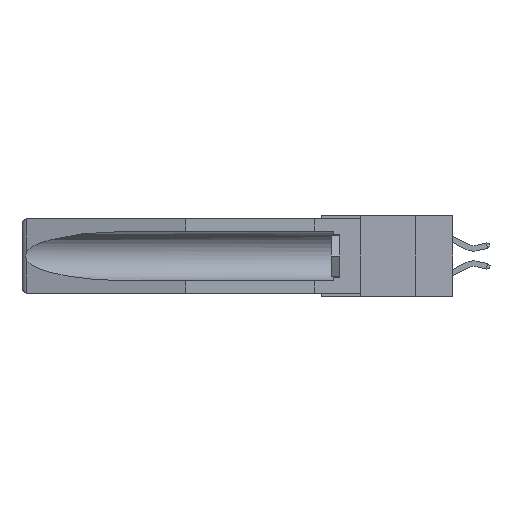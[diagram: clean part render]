
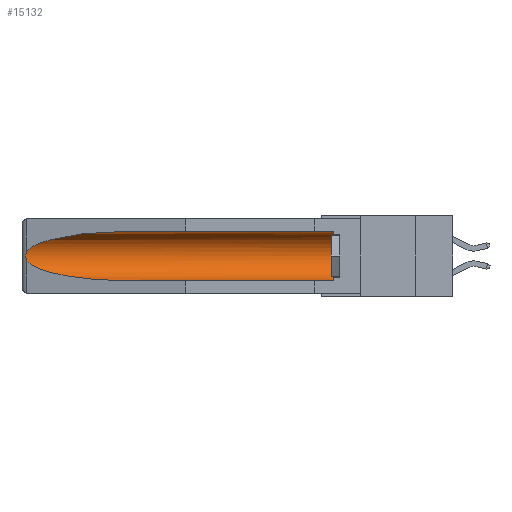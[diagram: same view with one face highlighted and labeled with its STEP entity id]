
A CAD part, left-side view. The second image highlights one B-rep face of the part: STEP entity #15132.
In plain terms, the highlighted cylindrical face has radius 2.857 mm (diameter 5.715 mm), a partial arc.
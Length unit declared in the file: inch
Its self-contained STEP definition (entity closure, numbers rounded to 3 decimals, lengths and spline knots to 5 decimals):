
#1424 = CARTESIAN_POINT ( 'NONE',  ( 0.26537, 1.52718, -0.14972 ) ) ;
#1479 = DIRECTION ( 'NONE',  ( 0., -1., 0. ) ) ;
#2629 = LINE ( 'NONE', #21175, #18509 ) ;
#2882 = CARTESIAN_POINT ( 'NONE',  ( 0.155, 1.07973, -0.284 ) ) ;
#3194 = VERTEX_POINT ( 'NONE', #13387 ) ;
#3253 = CARTESIAN_POINT ( 'NONE',  ( 0.155, 0.126, -0.059 ) ) ;
#4121 = ORIENTED_EDGE ( 'NONE', *, *, #8473, .T. ) ;
#4178 = ORIENTED_EDGE ( 'NONE', *, *, #28948, .T. ) ;
#4640 = CARTESIAN_POINT ( 'NONE',  ( 0.26537, 1.52718, -0.14972 ) ) ;
#5672 = CYLINDRICAL_SURFACE ( 'NONE', #25239, 0.1125 ) ;
#5760 = DIRECTION ( 'NONE',  ( 0., 1., 0. ) ) ;
#6600 = EDGE_CURVE ( 'NONE', #3194, #23858, #10625, .T. ) ;
#6605 = DIRECTION ( 'NONE',  ( 0., 1., 0. ) ) ;
#6966 = CARTESIAN_POINT ( 'NONE',  ( 0.26654, 1.53092, -0.15636 ) ) ;
#7737 =( BOUNDED_CURVE ( )  B_SPLINE_CURVE ( 3, ( #14965, #23502, #10684, #2882 ),
 .UNSPECIFIED., .F., .F. ) 
 B_SPLINE_CURVE_WITH_KNOTS ( ( 4, 4 ),
 ( 0.1948, 1.5708 ),
 .UNSPECIFIED. ) 
 CURVE ( )  GEOMETRIC_REPRESENTATION_ITEM ( )  RATIONAL_B_SPLINE_CURVE ( ( 1., 0.848, 0.848, 1. ) ) 
 REPRESENTATION_ITEM ( '' )  );
#8473 = EDGE_CURVE ( 'NONE', #30981, #20734, #12319, .T. ) ;
#9141 = CARTESIAN_POINT ( 'NONE',  ( 0.155, 0.126, -0.1715 ) ) ;
#9227 = ORIENTED_EDGE ( 'NONE', *, *, #21884, .F. ) ;
#9534 = CARTESIAN_POINT ( 'NONE',  ( 0.26655, 1.53094, -0.18657 ) ) ;
#9834 = CARTESIAN_POINT ( 'NONE',  ( 0.155, 1.07973, -0.059 ) ) ;
#10625 =( BOUNDED_CURVE ( )  B_SPLINE_CURVE ( 3, ( #9834, #17725, #25158, #4640 ),
 .UNSPECIFIED., .F., .F. ) 
 B_SPLINE_CURVE_WITH_KNOTS ( ( 4, 4 ),
 ( 4.71239, 6.08839 ),
 .UNSPECIFIED. ) 
 CURVE ( )  GEOMETRIC_REPRESENTATION_ITEM ( )  RATIONAL_B_SPLINE_CURVE ( ( 1., 0.848, 0.848, 1. ) ) 
 REPRESENTATION_ITEM ( '' )  );
#10684 = CARTESIAN_POINT ( 'NONE',  ( 0.21114, 1.30732, -0.284 ) ) ;
#11854 = CARTESIAN_POINT ( 'NONE',  ( 0.26537, 1.52718, -0.14972 ) ) ;
#11969 = VERTEX_POINT ( 'NONE', #20616 ) ;
#12319 = CIRCLE ( 'NONE', #31382, 0.1125 ) ;
#12494 = DIRECTION ( 'NONE',  ( 0., 1., 0. ) ) ;
#12590 = EDGE_LOOP ( 'NONE', ( #25673, #4178, #25975, #9227, #4121, #14475 ) ) ;
#13387 = CARTESIAN_POINT ( 'NONE',  ( 0.155, 1.07973, -0.059 ) ) ;
#14475 = ORIENTED_EDGE ( 'NONE', *, *, #19358, .T. ) ;
#14965 = CARTESIAN_POINT ( 'NONE',  ( 0.26537, 1.52718, -0.19328 ) ) ;
#15132 = ADVANCED_FACE ( 'NONE', ( #29536 ), #5672, .F. ) ;
#16653 = CARTESIAN_POINT ( 'NONE',  ( 0.155, 0.126, -0.284 ) ) ;
#16797 = LINE ( 'NONE', #27118, #26457 ) ;
#17076 = CARTESIAN_POINT ( 'NONE',  ( 0.2673, 1.53269, -0.17917 ) ) ;
#17725 = CARTESIAN_POINT ( 'NONE',  ( 0.21114, 1.30732, -0.059 ) ) ;
#18509 = VECTOR ( 'NONE', #5760, 39.37008 ) ;
#19358 = EDGE_CURVE ( 'NONE', #20734, #3194, #2629, .T. ) ;
#19470 = CARTESIAN_POINT ( 'NONE',  ( 0.2675, 1.53308, -0.16763 ) ) ;
#20616 = CARTESIAN_POINT ( 'NONE',  ( 0.26537, 1.52718, -0.19328 ) ) ;
#20734 = VERTEX_POINT ( 'NONE', #3253 ) ;
#21175 = CARTESIAN_POINT ( 'NONE',  ( 0.155, -0.30754, -0.059 ) ) ;
#21884 = EDGE_CURVE ( 'NONE', #30981, #28923, #16797, .T. ) ;
#22518 = DIRECTION ( 'NONE',  ( 0., 0., 1. ) ) ;
#23502 = CARTESIAN_POINT ( 'NONE',  ( 0.25451, 1.48313, -0.24835 ) ) ;
#23858 = VERTEX_POINT ( 'NONE', #11854 ) ;
#24739 = CARTESIAN_POINT ( 'NONE',  ( 0.26537, 1.52718, -0.19328 ) ) ;
#24972 = CARTESIAN_POINT ( 'NONE',  ( 0.2675, 1.53308, -0.17534 ) ) ;
#25158 = CARTESIAN_POINT ( 'NONE',  ( 0.25451, 1.48313, -0.09465 ) ) ;
#25239 = AXIS2_PLACEMENT_3D ( 'NONE', #27962, #12494, #30553 ) ;
#25673 = ORIENTED_EDGE ( 'NONE', *, *, #6600, .T. ) ;
#25975 = ORIENTED_EDGE ( 'NONE', *, *, #27545, .T. ) ;
#26457 = VECTOR ( 'NONE', #6605, 39.37008 ) ;
#27118 = CARTESIAN_POINT ( 'NONE',  ( 0.155, -0.30754, -0.284 ) ) ;
#27545 = EDGE_CURVE ( 'NONE', #11969, #28923, #7737, .T. ) ;
#27584 = CARTESIAN_POINT ( 'NONE',  ( 0.155, 1.07973, -0.284 ) ) ;
#27785 = B_SPLINE_CURVE_WITH_KNOTS ( 'NONE', 3,
 ( #1424, #29957, #6966, #32824, #19470, #24972, #17076, #9534, #30180, #24739 ),
 .UNSPECIFIED., .F., .F.,
 ( 4, 2, 2, 2, 4 ),
 ( 0., 0.00029, 0.00058, 0.00087, 0.00117 ),
 .UNSPECIFIED. ) ;
#27962 = CARTESIAN_POINT ( 'NONE',  ( 0.155, -0.30754, -0.1715 ) ) ;
#28923 = VERTEX_POINT ( 'NONE', #27584 ) ;
#28948 = EDGE_CURVE ( 'NONE', #23858, #11969, #27785, .T. ) ;
#29536 = FACE_OUTER_BOUND ( 'NONE', #12590, .T. ) ;
#29957 = CARTESIAN_POINT ( 'NONE',  ( 0.26597, 1.52961, -0.15275 ) ) ;
#30180 = CARTESIAN_POINT ( 'NONE',  ( 0.26597, 1.5296, -0.19026 ) ) ;
#30553 = DIRECTION ( 'NONE',  ( 0., 0., 1. ) ) ;
#30981 = VERTEX_POINT ( 'NONE', #16653 ) ;
#31382 = AXIS2_PLACEMENT_3D ( 'NONE', #9141, #1479, #22518 ) ;
#32824 = CARTESIAN_POINT ( 'NONE',  ( 0.2673, 1.5327, -0.16383 ) ) ;
